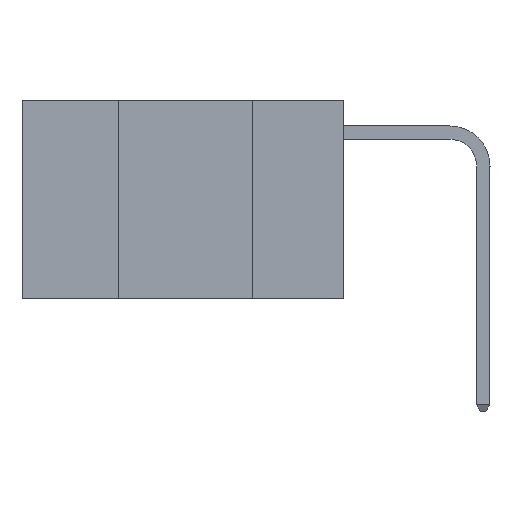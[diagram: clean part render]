
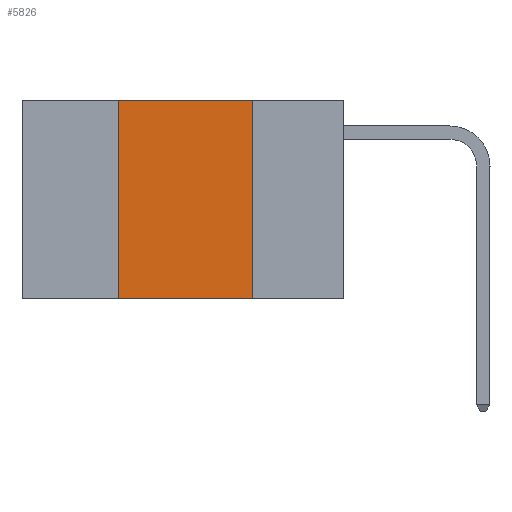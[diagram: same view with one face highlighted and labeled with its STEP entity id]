
A CAD part, left-side view. The second image highlights one B-rep face of the part: STEP entity #5826.
In plain terms, the highlighted planar face has unit normal (-1, 0, 0).
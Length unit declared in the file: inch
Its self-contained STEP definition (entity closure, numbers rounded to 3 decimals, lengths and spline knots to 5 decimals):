
#230 = VERTEX_POINT ( 'NONE', #4753 ) ;
#385 = DIRECTION ( 'NONE',  ( 1., 0., 0. ) ) ;
#422 = ORIENTED_EDGE ( 'NONE', *, *, #8068, .F. ) ;
#663 = CARTESIAN_POINT ( 'NONE',  ( 0., 0.42, 0. ) ) ;
#740 = ORIENTED_EDGE ( 'NONE', *, *, #3968, .F. ) ;
#1286 = CARTESIAN_POINT ( 'NONE',  ( 0., 0.42, -0.37 ) ) ;
#3303 = CARTESIAN_POINT ( 'NONE',  ( 0., 0.6, 0. ) ) ;
#3314 = VERTEX_POINT ( 'NONE', #1286 ) ;
#3499 = ORIENTED_EDGE ( 'NONE', *, *, #8141, .F. ) ;
#3651 = CARTESIAN_POINT ( 'NONE',  ( 0., 0.17, 0. ) ) ;
#3885 = LINE ( 'NONE', #663, #11476 ) ;
#3968 = EDGE_CURVE ( 'NONE', #12802, #230, #4898, .T. ) ;
#4389 = VERTEX_POINT ( 'NONE', #6064 ) ;
#4753 = CARTESIAN_POINT ( 'NONE',  ( 0., 0.17, 0. ) ) ;
#4898 = LINE ( 'NONE', #3303, #12704 ) ;
#5318 = DIRECTION ( 'NONE',  ( 0., -1., 0. ) ) ;
#5513 = PLANE ( 'NONE',  #6727 ) ;
#5826 = ADVANCED_FACE ( 'NONE', ( #12386 ), #5513, .F. ) ;
#6064 = CARTESIAN_POINT ( 'NONE',  ( 0., 0.17, -0.37 ) ) ;
#6213 = ORIENTED_EDGE ( 'NONE', *, *, #8492, .T. ) ;
#6727 = AXIS2_PLACEMENT_3D ( 'NONE', #12341, #385, #7550 ) ;
#6900 = VECTOR ( 'NONE', #5318, 39.37008 ) ;
#7212 = LINE ( 'NONE', #9325, #6900 ) ;
#7228 = VECTOR ( 'NONE', #11563, 39.37008 ) ;
#7536 = LINE ( 'NONE', #3651, #7228 ) ;
#7550 = DIRECTION ( 'NONE',  ( 0., 0., -1. ) ) ;
#7951 = EDGE_LOOP ( 'NONE', ( #422, #740, #3499, #6213 ) ) ;
#8068 = EDGE_CURVE ( 'NONE', #230, #4389, #7536, .T. ) ;
#8141 = EDGE_CURVE ( 'NONE', #3314, #12802, #3885, .T. ) ;
#8492 = EDGE_CURVE ( 'NONE', #3314, #4389, #7212, .T. ) ;
#9215 = CARTESIAN_POINT ( 'NONE',  ( 0., 0.42, 0. ) ) ;
#9325 = CARTESIAN_POINT ( 'NONE',  ( 0., 0.6, -0.37 ) ) ;
#9346 = DIRECTION ( 'NONE',  ( 0., -1., 0. ) ) ;
#10740 = DIRECTION ( 'NONE',  ( 0., 0., 1. ) ) ;
#11476 = VECTOR ( 'NONE', #10740, 39.37008 ) ;
#11563 = DIRECTION ( 'NONE',  ( 0., 0., -1. ) ) ;
#12341 = CARTESIAN_POINT ( 'NONE',  ( 0., 0.6, 0. ) ) ;
#12386 = FACE_OUTER_BOUND ( 'NONE', #7951, .T. ) ;
#12704 = VECTOR ( 'NONE', #9346, 39.37008 ) ;
#12802 = VERTEX_POINT ( 'NONE', #9215 ) ;
